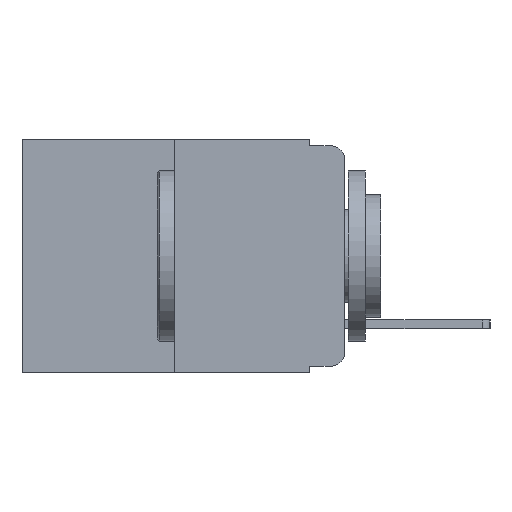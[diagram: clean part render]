
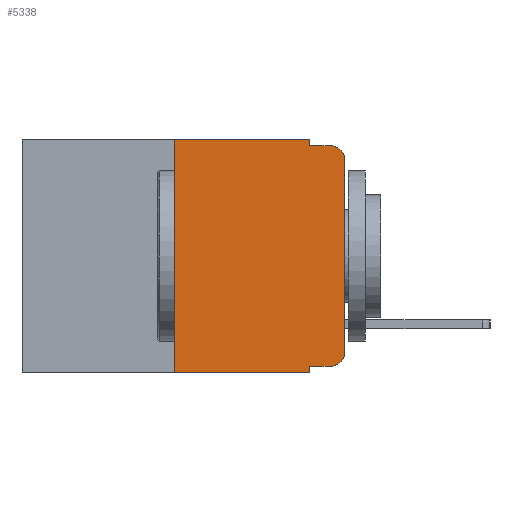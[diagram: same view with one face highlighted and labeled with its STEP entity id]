
A CAD part, left-side view. The second image highlights one B-rep face of the part: STEP entity #5338.
In plain terms, the highlighted planar face has unit normal (-1, 0, 0).
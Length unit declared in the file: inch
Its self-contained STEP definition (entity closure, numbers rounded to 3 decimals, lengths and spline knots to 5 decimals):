
#175 = ORIENTED_EDGE ( 'NONE', *, *, #2137, .F. ) ;
#306 = CIRCLE ( 'NONE', #9290, 0.02 ) ;
#568 = ORIENTED_EDGE ( 'NONE', *, *, #882, .T. ) ;
#611 = ORIENTED_EDGE ( 'NONE', *, *, #5774, .T. ) ;
#882 = EDGE_CURVE ( 'NONE', #3881, #2177, #8564, .T. ) ;
#1157 = CARTESIAN_POINT ( 'NONE',  ( 0., 0.02, -0.01 ) ) ;
#1615 = ORIENTED_EDGE ( 'NONE', *, *, #21132, .T. ) ;
#1641 = ORIENTED_EDGE ( 'NONE', *, *, #11025, .T. ) ;
#1717 = CARTESIAN_POINT ( 'NONE',  ( 0., 0.051, 0. ) ) ;
#1765 = ORIENTED_EDGE ( 'NONE', *, *, #20309, .F. ) ;
#2137 = EDGE_CURVE ( 'NONE', #3881, #13189, #15691, .T. ) ;
#2177 = VERTEX_POINT ( 'NONE', #19584 ) ;
#2233 = ORIENTED_EDGE ( 'NONE', *, *, #22617, .F. ) ;
#2494 = EDGE_LOOP ( 'NONE', ( #1615, #1641, #1765, #2233, #3216, #3692, #11549, #175, #568, #611 ) ) ;
#3149 = CARTESIAN_POINT ( 'NONE',  ( 0., 0.473, 0. ) ) ;
#3216 = ORIENTED_EDGE ( 'NONE', *, *, #17572, .F. ) ;
#3434 = DIRECTION ( 'NONE',  ( 1., 0., 0. ) ) ;
#3534 = CIRCLE ( 'NONE', #21050, 0.02 ) ;
#3557 = FACE_OUTER_BOUND ( 'NONE', #2494, .T. ) ;
#3680 = CARTESIAN_POINT ( 'NONE',  ( 0., 0.25, -0.343 ) ) ;
#3692 = ORIENTED_EDGE ( 'NONE', *, *, #21475, .F. ) ;
#3713 = DIRECTION ( 'NONE',  ( 0., -1., 0. ) ) ;
#3881 = VERTEX_POINT ( 'NONE', #15656 ) ;
#4410 = LINE ( 'NONE', #11233, #22503 ) ;
#4711 = VERTEX_POINT ( 'NONE', #1157 ) ;
#5061 = DIRECTION ( 'NONE',  ( 0., 0., -1. ) ) ;
#5329 = LINE ( 'NONE', #15988, #18791 ) ;
#5338 = ADVANCED_FACE ( 'NONE', ( #3557 ), #7278, .F. ) ;
#5737 = DIRECTION ( 'NONE',  ( 0., 0., -1. ) ) ;
#5774 = EDGE_CURVE ( 'NONE', #2177, #7835, #3534, .T. ) ;
#5998 = VERTEX_POINT ( 'NONE', #3680 ) ;
#6101 = VECTOR ( 'NONE', #6850, 39.37008 ) ;
#6264 = DIRECTION ( 'NONE',  ( -1., 0., 0. ) ) ;
#6850 = DIRECTION ( 'NONE',  ( 0., 0., 1. ) ) ;
#7278 = PLANE ( 'NONE',  #13392 ) ;
#7361 = CARTESIAN_POINT ( 'NONE',  ( 0., 0.051, 0. ) ) ;
#7767 = CARTESIAN_POINT ( 'NONE',  ( 0., 0.25, 0. ) ) ;
#7835 = VERTEX_POINT ( 'NONE', #21417 ) ;
#8463 = DIRECTION ( 'NONE',  ( -1., 0., 0. ) ) ;
#8564 = LINE ( 'NONE', #22502, #21387 ) ;
#8627 = DIRECTION ( 'NONE',  ( 0., -1., 0. ) ) ;
#8631 = CARTESIAN_POINT ( 'NONE',  ( 0., 0.25, 0. ) ) ;
#9190 = VECTOR ( 'NONE', #19881, 39.37008 ) ;
#9290 = AXIS2_PLACEMENT_3D ( 'NONE', #16817, #6264, #18557 ) ;
#10226 = VECTOR ( 'NONE', #3713, 39.37008 ) ;
#10795 = LINE ( 'NONE', #14368, #10226 ) ;
#11025 = EDGE_CURVE ( 'NONE', #19305, #4711, #306, .T. ) ;
#11045 = VECTOR ( 'NONE', #5737, 39.37008 ) ;
#11233 = CARTESIAN_POINT ( 'NONE',  ( 0., 0.051, 0. ) ) ;
#11549 = ORIENTED_EDGE ( 'NONE', *, *, #20482, .T. ) ;
#11954 = VERTEX_POINT ( 'NONE', #7361 ) ;
#13189 = VERTEX_POINT ( 'NONE', #17808 ) ;
#13391 = VERTEX_POINT ( 'NONE', #18321 ) ;
#13392 = AXIS2_PLACEMENT_3D ( 'NONE', #3149, #3434, #5061 ) ;
#13913 = LINE ( 'NONE', #19804, #9190 ) ;
#14288 = DIRECTION ( 'NONE',  ( 0., -1., 0. ) ) ;
#14368 = CARTESIAN_POINT ( 'NONE',  ( 0., 0.473, 0. ) ) ;
#14706 = DIRECTION ( 'NONE',  ( 0., 0., -1. ) ) ;
#15500 = LINE ( 'NONE', #8631, #6101 ) ;
#15627 = CARTESIAN_POINT ( 'NONE',  ( 0., 0.051, -0.01 ) ) ;
#15656 = CARTESIAN_POINT ( 'NONE',  ( 0., 0.051, -0.333 ) ) ;
#15691 = LINE ( 'NONE', #1717, #11045 ) ;
#15988 = CARTESIAN_POINT ( 'NONE',  ( 0., 0.473, -0.343 ) ) ;
#16817 = CARTESIAN_POINT ( 'NONE',  ( 0., 0.02, -0.03 ) ) ;
#17465 = VECTOR ( 'NONE', #8627, 39.37008 ) ;
#17572 = EDGE_CURVE ( 'NONE', #18200, #11954, #10795, .T. ) ;
#17808 = CARTESIAN_POINT ( 'NONE',  ( 0., 0.051, -0.343 ) ) ;
#17916 = CARTESIAN_POINT ( 'NONE',  ( 0., 0., -0.03 ) ) ;
#18200 = VERTEX_POINT ( 'NONE', #7767 ) ;
#18321 = CARTESIAN_POINT ( 'NONE',  ( 0., 0.051, -0.01 ) ) ;
#18557 = DIRECTION ( 'NONE',  ( 0., 0., -1. ) ) ;
#18791 = VECTOR ( 'NONE', #14288, 39.37008 ) ;
#18918 = CARTESIAN_POINT ( 'NONE',  ( 0., 0.02, -0.313 ) ) ;
#19305 = VERTEX_POINT ( 'NONE', #17916 ) ;
#19584 = CARTESIAN_POINT ( 'NONE',  ( 0., 0.02, -0.333 ) ) ;
#19804 = CARTESIAN_POINT ( 'NONE',  ( 0., 0., 0. ) ) ;
#19881 = DIRECTION ( 'NONE',  ( 0., 0., 1. ) ) ;
#20309 = EDGE_CURVE ( 'NONE', #13391, #4711, #22048, .T. ) ;
#20482 = EDGE_CURVE ( 'NONE', #5998, #13189, #5329, .T. ) ;
#20674 = DIRECTION ( 'NONE',  ( 0., 0., -1. ) ) ;
#21050 = AXIS2_PLACEMENT_3D ( 'NONE', #18918, #8463, #20674 ) ;
#21132 = EDGE_CURVE ( 'NONE', #7835, #19305, #13913, .T. ) ;
#21387 = VECTOR ( 'NONE', #21638, 39.37008 ) ;
#21417 = CARTESIAN_POINT ( 'NONE',  ( 0., 0., -0.313 ) ) ;
#21475 = EDGE_CURVE ( 'NONE', #5998, #18200, #15500, .T. ) ;
#21638 = DIRECTION ( 'NONE',  ( 0., -1., 0. ) ) ;
#22048 = LINE ( 'NONE', #15627, #17465 ) ;
#22502 = CARTESIAN_POINT ( 'NONE',  ( 0., 0.051, -0.333 ) ) ;
#22503 = VECTOR ( 'NONE', #14706, 39.37008 ) ;
#22617 = EDGE_CURVE ( 'NONE', #11954, #13391, #4410, .T. ) ;
